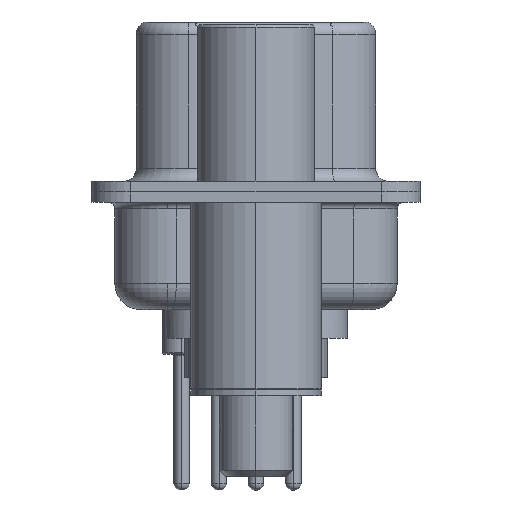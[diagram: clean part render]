
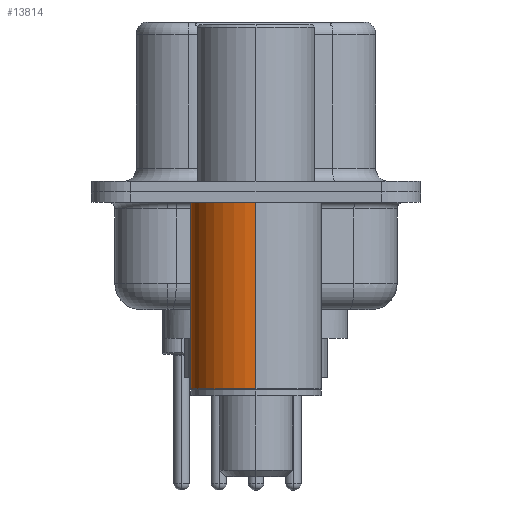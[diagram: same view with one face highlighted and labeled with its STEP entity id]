
A CAD part, left-side view. The second image highlights one B-rep face of the part: STEP entity #13814.
In plain terms, the highlighted cylindrical face has radius 2.5 mm (diameter 5 mm), a partial arc.
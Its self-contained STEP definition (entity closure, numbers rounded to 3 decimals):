
#299 = ORIENTED_EDGE ( 'NONE', *, *, #13752, .T. ) ;
#708 = CIRCLE ( 'NONE', #4402, 2.5 ) ;
#947 = CARTESIAN_POINT ( 'NONE',  ( 0., 0., 0.581 ) ) ;
#1419 = DIRECTION ( 'NONE',  ( 0., 0., 1. ) ) ;
#2331 = EDGE_LOOP ( 'NONE', ( #299, #5557, #20226, #11887 ) ) ;
#3043 = AXIS2_PLACEMENT_3D ( 'NONE', #947, #1419, #13423 ) ;
#3399 = CARTESIAN_POINT ( 'NONE',  ( -2.5, 0., -0.4 ) ) ;
#3909 = VECTOR ( 'NONE', #7160, 1000. ) ;
#4174 = DIRECTION ( 'NONE',  ( 0., 0., 1. ) ) ;
#4402 = AXIS2_PLACEMENT_3D ( 'NONE', #8790, #20849, #10535 ) ;
#4491 = CARTESIAN_POINT ( 'NONE',  ( -2.5, 0., -7.525 ) ) ;
#4628 = EDGE_CURVE ( 'NONE', #13252, #7040, #12815, .T. ) ;
#5557 = ORIENTED_EDGE ( 'NONE', *, *, #4628, .T. ) ;
#5685 = CARTESIAN_POINT ( 'NONE',  ( 2.5, 0., -0.4 ) ) ;
#6114 = EDGE_CURVE ( 'NONE', #16760, #14807, #6539, .T. ) ;
#6539 = LINE ( 'NONE', #17102, #14140 ) ;
#6653 = CYLINDRICAL_SURFACE ( 'NONE', #3043, 2.5 ) ;
#6757 = DIRECTION ( 'NONE',  ( 0., 0., 1. ) ) ;
#7040 = VERTEX_POINT ( 'NONE', #3399 ) ;
#7160 = DIRECTION ( 'NONE',  ( 0., 0., 1. ) ) ;
#7357 = CARTESIAN_POINT ( 'NONE',  ( -2.5, 0., 0.581 ) ) ;
#8790 = CARTESIAN_POINT ( 'NONE',  ( 0., 0., -0.4 ) ) ;
#10535 = DIRECTION ( 'NONE',  ( 1., 0., 0. ) ) ;
#11887 = ORIENTED_EDGE ( 'NONE', *, *, #6114, .F. ) ;
#12815 = LINE ( 'NONE', #7357, #3909 ) ;
#13252 = VERTEX_POINT ( 'NONE', #4491 ) ;
#13423 = DIRECTION ( 'NONE',  ( 1., 0., 0. ) ) ;
#13752 = EDGE_CURVE ( 'NONE', #16760, #13252, #17474, .T. ) ;
#13814 = ADVANCED_FACE ( 'NONE', ( #15886 ), #6653, .T. ) ;
#14140 = VECTOR ( 'NONE', #6757, 1000. ) ;
#14549 = CARTESIAN_POINT ( 'NONE',  ( 0., 0., -7.525 ) ) ;
#14807 = VERTEX_POINT ( 'NONE', #5685 ) ;
#15886 = FACE_OUTER_BOUND ( 'NONE', #2331, .T. ) ;
#16280 = DIRECTION ( 'NONE',  ( 1., 0., 0. ) ) ;
#16760 = VERTEX_POINT ( 'NONE', #17251 ) ;
#16790 = EDGE_CURVE ( 'NONE', #14807, #7040, #708, .T. ) ;
#17102 = CARTESIAN_POINT ( 'NONE',  ( 2.5, 0., 0.581 ) ) ;
#17251 = CARTESIAN_POINT ( 'NONE',  ( 2.5, 0., -7.525 ) ) ;
#17474 = CIRCLE ( 'NONE', #18491, 2.5 ) ;
#18491 = AXIS2_PLACEMENT_3D ( 'NONE', #14549, #4174, #16280 ) ;
#20226 = ORIENTED_EDGE ( 'NONE', *, *, #16790, .F. ) ;
#20849 = DIRECTION ( 'NONE',  ( 0., 0., 1. ) ) ;
